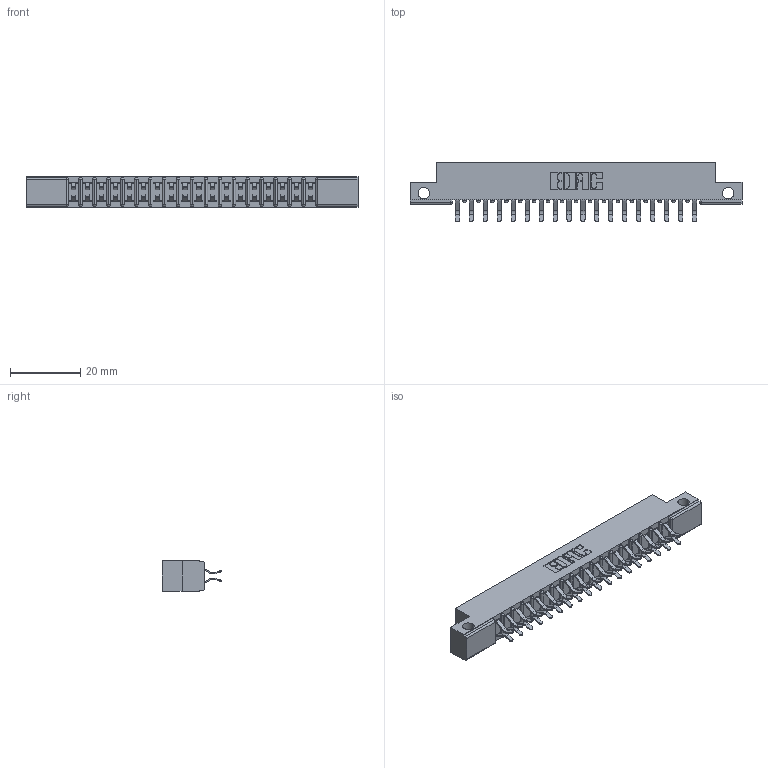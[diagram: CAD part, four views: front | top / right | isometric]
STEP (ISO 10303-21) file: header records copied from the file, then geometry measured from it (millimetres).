
FILE_DESCRIPTION (( 'STEP AP203' ), '1' );
FILE_NAME ('357-036-456-212.STEP', '2020-10-03T18:04:38', ( '' ), ( '' ), 'SwSTEP 2.0', 'SolidWorks 2020', '' );
FILE_SCHEMA (( 'CONFIG_CONTROL_DESIGN' ));
Length unit declared in the file: inch
Products named in the file (3): 307-290-001_556; 357-036-456-212; 307 Part_.128 Dia Side Mounting Holes
Assembly tree (37 placements, depth 2):
  357-036-456-212
    307 Part_.128 Dia Side Mounting Holes
    307-290-001_556  x36
Bounding box: 94.34 x 16.97 x 8.71 mm (x, y, z)
Volume: 6088.6 mm3; surface area: 10371 mm2
Topology: 37 solids, 37 shells, 1937 faces, 5435 edges, 3522 vertices
Faces by surface type: plane 1258, cylinder 641, sphere 38
Entity records: 19072 total; most frequent: CARTESIAN_POINT 3126, ORIENTED_EDGE 3094, DIRECTION 3073, EDGE_CURVE 1547, VECTOR 1175, LINE 1175, VERTEX_POINT 1002, AXIS2_PLACEMENT_3D 949
